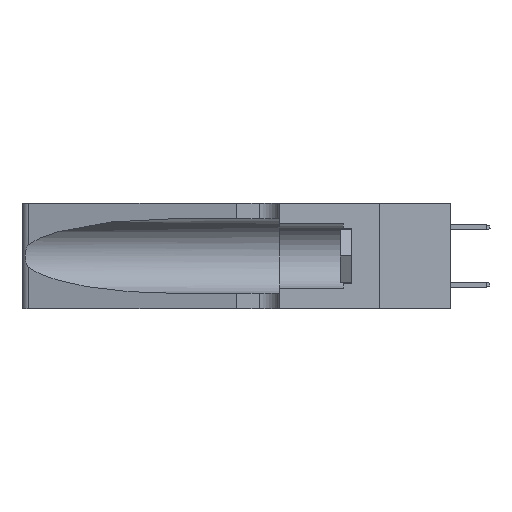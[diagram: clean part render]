
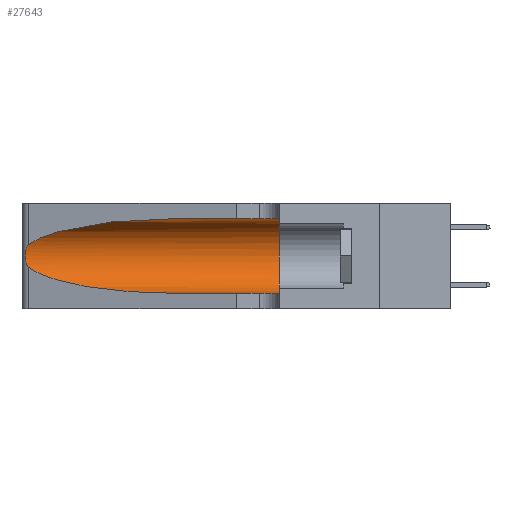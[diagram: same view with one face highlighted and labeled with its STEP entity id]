
A CAD part, left-side view. The second image highlights one B-rep face of the part: STEP entity #27643.
In plain terms, the highlighted cylindrical face has radius 3.308 mm (diameter 6.617 mm), a partial arc.
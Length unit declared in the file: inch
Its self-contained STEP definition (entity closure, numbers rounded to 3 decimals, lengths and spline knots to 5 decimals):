
#479 = CARTESIAN_POINT ( 'NONE',  ( 0.1305, 0.72297, 0.05475 ) ) ;
#1885 = DIRECTION ( 'NONE',  ( 0., -1., 0. ) ) ;
#2317 = CARTESIAN_POINT ( 'NONE',  ( 0.18966, 0.96281, 0.31525 ) ) ;
#2500 =( BOUNDED_CURVE ( )  B_SPLINE_CURVE ( 3, ( #35306, #2317, #28102, #42749 ),
 .UNSPECIFIED., .F., .F. ) 
 B_SPLINE_CURVE_WITH_KNOTS ( ( 4, 4 ),
 ( 1.5708, 2.84003 ),
 .UNSPECIFIED. ) 
 CURVE ( )  GEOMETRIC_REPRESENTATION_ITEM ( )  RATIONAL_B_SPLINE_CURVE ( ( 1., 0.87, 0.87, 1. ) ) 
 REPRESENTATION_ITEM ( '' )  );
#3295 = ORIENTED_EDGE ( 'NONE', *, *, #14049, .T. ) ;
#3473 = LINE ( 'NONE', #39589, #34357 ) ;
#4142 = DIRECTION ( 'NONE',  ( 0., 0., -1. ) ) ;
#4458 = VERTEX_POINT ( 'NONE', #12391 ) ;
#5224 = CARTESIAN_POINT ( 'NONE',  ( 0.25487, 1.22718, 0.22369 ) ) ;
#5692 = CARTESIAN_POINT ( 'NONE',  ( 0.26075, 1.23896, 0.19203 ) ) ;
#7515 = CYLINDRICAL_SURFACE ( 'NONE', #38635, 0.13025 ) ;
#8516 = EDGE_LOOP ( 'NONE', ( #30686, #31077, #3295, #45343, #29794, #45767 ) ) ;
#9054 = CARTESIAN_POINT ( 'NONE',  ( 0.25639, 1.23186, 0.15144 ) ) ;
#9123 = CARTESIAN_POINT ( 'NONE',  ( 0.2373, 1.15595, 0.08982 ) ) ;
#9279 = CARTESIAN_POINT ( 'NONE',  ( 0.25555, 1.22993, 0.14849 ) ) ;
#9516 = CARTESIAN_POINT ( 'NONE',  ( 0.25789, 1.23486, 0.15765 ) ) ;
#10070 = EDGE_CURVE ( 'NONE', #13863, #37559, #3473, .T. ) ;
#11608 = FACE_OUTER_BOUND ( 'NONE', #8516, .T. ) ;
#12391 = CARTESIAN_POINT ( 'NONE',  ( 0.25487, 1.22718, 0.22369 ) ) ;
#12669 = CARTESIAN_POINT ( 'NONE',  ( 0.26018, 1.23835, 0.19895 ) ) ;
#13863 = VERTEX_POINT ( 'NONE', #479 ) ;
#14049 = EDGE_CURVE ( 'NONE', #25688, #13863, #45266, .T. ) ;
#14352 = EDGE_CURVE ( 'NONE', #45916, #37559, #41584, .T. ) ;
#14783 = DIRECTION ( 'NONE',  ( 0., -1., 0. ) ) ;
#15793 = CARTESIAN_POINT ( 'NONE',  ( 0.25856, 1.23593, 0.16098 ) ) ;
#16747 = CARTESIAN_POINT ( 'NONE',  ( 0.25555, 1.22994, 0.2215 ) ) ;
#17048 = CARTESIAN_POINT ( 'NONE',  ( 0.1305, 0.72297, 0.05475 ) ) ;
#17278 = LINE ( 'NONE', #38717, #32967 ) ;
#18100 = CARTESIAN_POINT ( 'NONE',  ( 0.1305, 1.61858, 0.185 ) ) ;
#19952 = EDGE_CURVE ( 'NONE', #37250, #4458, #2500, .T. ) ;
#20370 = CARTESIAN_POINT ( 'NONE',  ( 0.1305, 0.35, 0.05475 ) ) ;
#22211 = DIRECTION ( 'NONE',  ( 0., -1., 0. ) ) ;
#23761 = CARTESIAN_POINT ( 'NONE',  ( 0.25487, 1.22718, 0.14631 ) ) ;
#24224 = CARTESIAN_POINT ( 'NONE',  ( 0.25639, 1.23184, 0.21858 ) ) ;
#24288 = CARTESIAN_POINT ( 'NONE',  ( 0.18966, 0.96281, 0.05475 ) ) ;
#25247 = CARTESIAN_POINT ( 'NONE',  ( 0.1305, 0.72297, 0.31525 ) ) ;
#25688 = VERTEX_POINT ( 'NONE', #25741 ) ;
#25741 = CARTESIAN_POINT ( 'NONE',  ( 0.25487, 1.22718, 0.14631 ) ) ;
#26997 = AXIS2_PLACEMENT_3D ( 'NONE', #34797, #30941, #35035 ) ;
#27376 = CARTESIAN_POINT ( 'NONE',  ( 0.26075, 1.23896, 0.178 ) ) ;
#27643 = ADVANCED_FACE ( 'NONE', ( #11608 ), #7515, .F. ) ;
#27844 = CARTESIAN_POINT ( 'NONE',  ( 0.25787, 1.23484, 0.2124 ) ) ;
#27911 = CARTESIAN_POINT ( 'NONE',  ( 0.25487, 1.22718, 0.14631 ) ) ;
#28102 = CARTESIAN_POINT ( 'NONE',  ( 0.2373, 1.15595, 0.28018 ) ) ;
#29794 = ORIENTED_EDGE ( 'NONE', *, *, #14352, .F. ) ;
#30686 = ORIENTED_EDGE ( 'NONE', *, *, #19952, .T. ) ;
#30941 = DIRECTION ( 'NONE',  ( 0., 1., 0. ) ) ;
#31077 = ORIENTED_EDGE ( 'NONE', *, *, #34949, .T. ) ;
#32967 = VECTOR ( 'NONE', #1885, 39.37008 ) ;
#33556 = B_SPLINE_CURVE_WITH_KNOTS ( 'NONE', 3,
 ( #5224, #16747, #24224, #27844, #45651, #12669, #5692, #27376, #42037, #15793, #9516, #9054, #9279, #23761 ),
 .UNSPECIFIED., .F., .F.,
 ( 4, 2, 2, 2, 2, 2, 4 ),
 ( 0., 0.00027, 0.00053, 0.00107, 0.0016, 0.00187, 0.00214 ),
 .UNSPECIFIED. ) ;
#34357 = VECTOR ( 'NONE', #14783, 39.37008 ) ;
#34797 = CARTESIAN_POINT ( 'NONE',  ( 0.1305, 0.35, 0.185 ) ) ;
#34949 = EDGE_CURVE ( 'NONE', #4458, #25688, #33556, .T. ) ;
#35035 = DIRECTION ( 'NONE',  ( 0., 0., 1. ) ) ;
#35306 = CARTESIAN_POINT ( 'NONE',  ( 0.1305, 0.72297, 0.31525 ) ) ;
#37025 = EDGE_CURVE ( 'NONE', #37250, #45916, #17278, .T. ) ;
#37250 = VERTEX_POINT ( 'NONE', #25247 ) ;
#37559 = VERTEX_POINT ( 'NONE', #20370 ) ;
#38635 = AXIS2_PLACEMENT_3D ( 'NONE', #18100, #22211, #4142 ) ;
#38717 = CARTESIAN_POINT ( 'NONE',  ( 0.1305, 1.61858, 0.31525 ) ) ;
#39589 = CARTESIAN_POINT ( 'NONE',  ( 0.1305, 1.61858, 0.05475 ) ) ;
#41584 = CIRCLE ( 'NONE', #26997, 0.13025 ) ;
#42037 = CARTESIAN_POINT ( 'NONE',  ( 0.26017, 1.23833, 0.17102 ) ) ;
#42749 = CARTESIAN_POINT ( 'NONE',  ( 0.25487, 1.22718, 0.22369 ) ) ;
#45266 =( BOUNDED_CURVE ( )  B_SPLINE_CURVE ( 3, ( #27911, #9123, #24288, #17048 ),
 .UNSPECIFIED., .F., .F. ) 
 B_SPLINE_CURVE_WITH_KNOTS ( ( 4, 4 ),
 ( 3.44316, 4.71239 ),
 .UNSPECIFIED. ) 
 CURVE ( )  GEOMETRIC_REPRESENTATION_ITEM ( )  RATIONAL_B_SPLINE_CURVE ( ( 1., 0.87, 0.87, 1. ) ) 
 REPRESENTATION_ITEM ( '' )  );
#45343 = ORIENTED_EDGE ( 'NONE', *, *, #10070, .T. ) ;
#45651 = CARTESIAN_POINT ( 'NONE',  ( 0.25854, 1.2359, 0.20912 ) ) ;
#45767 = ORIENTED_EDGE ( 'NONE', *, *, #37025, .F. ) ;
#45916 = VERTEX_POINT ( 'NONE', #46177 ) ;
#46177 = CARTESIAN_POINT ( 'NONE',  ( 0.1305, 0.35, 0.31525 ) ) ;
